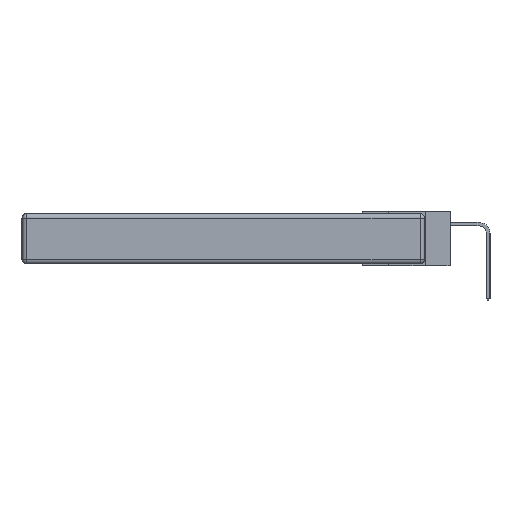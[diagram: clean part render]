
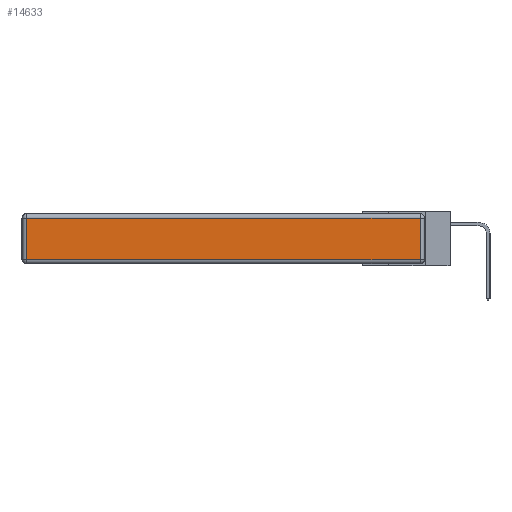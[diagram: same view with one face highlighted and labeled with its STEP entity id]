
A CAD part, left-side view. The second image highlights one B-rep face of the part: STEP entity #14633.
In plain terms, the highlighted planar face has unit normal (-1, 0, 0).
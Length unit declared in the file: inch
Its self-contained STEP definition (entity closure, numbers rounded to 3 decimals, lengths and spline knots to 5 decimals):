
#214 = VERTEX_POINT ( 'NONE', #12828 ) ;
#379 = VERTEX_POINT ( 'NONE', #14733 ) ;
#755 = CARTESIAN_POINT ( 'NONE',  ( 0., 0., -0.313 ) ) ;
#1602 = DIRECTION ( 'NONE',  ( 0., 0., 1. ) ) ;
#2339 = EDGE_CURVE ( 'NONE', #214, #11328, #6096, .T. ) ;
#2449 = ORIENTED_EDGE ( 'NONE', *, *, #2339, .T. ) ;
#4370 = ORIENTED_EDGE ( 'NONE', *, *, #13561, .T. ) ;
#4635 = CARTESIAN_POINT ( 'NONE',  ( 0., 2.75, -0.03 ) ) ;
#6096 = LINE ( 'NONE', #17140, #16647 ) ;
#6126 = DIRECTION ( 'NONE',  ( 0., 0., -1. ) ) ;
#6571 = EDGE_CURVE ( 'NONE', #11328, #15011, #13631, .T. ) ;
#7187 = LINE ( 'NONE', #755, #8609 ) ;
#8020 = LINE ( 'NONE', #10460, #13421 ) ;
#8609 = VECTOR ( 'NONE', #14174, 39.37008 ) ;
#8952 = PLANE ( 'NONE',  #14220 ) ;
#9054 = CARTESIAN_POINT ( 'NONE',  ( 0., 0.03, -0.03 ) ) ;
#9295 = FACE_OUTER_BOUND ( 'NONE', #10031, .T. ) ;
#9545 = DIRECTION ( 'NONE',  ( 0., 0., 1. ) ) ;
#10031 = EDGE_LOOP ( 'NONE', ( #4370, #2449, #17600, #19338 ) ) ;
#10460 = CARTESIAN_POINT ( 'NONE',  ( 0., 2.72, -0.343 ) ) ;
#11328 = VERTEX_POINT ( 'NONE', #9054 ) ;
#12049 = DIRECTION ( 'NONE',  ( -1., 0., 0. ) ) ;
#12061 = DIRECTION ( 'NONE',  ( 0., 1., 0. ) ) ;
#12828 = CARTESIAN_POINT ( 'NONE',  ( 0., 0.03, -0.313 ) ) ;
#13421 = VECTOR ( 'NONE', #6126, 39.37008 ) ;
#13492 = CARTESIAN_POINT ( 'NONE',  ( 0., 0., -0.343 ) ) ;
#13561 = EDGE_CURVE ( 'NONE', #379, #214, #7187, .T. ) ;
#13631 = LINE ( 'NONE', #4635, #16951 ) ;
#14174 = DIRECTION ( 'NONE',  ( 0., -1., 0. ) ) ;
#14220 = AXIS2_PLACEMENT_3D ( 'NONE', #13492, #12049, #1602 ) ;
#14633 = ADVANCED_FACE ( 'NONE', ( #9295 ), #8952, .T. ) ;
#14733 = CARTESIAN_POINT ( 'NONE',  ( 0., 2.72, -0.313 ) ) ;
#15011 = VERTEX_POINT ( 'NONE', #18201 ) ;
#16647 = VECTOR ( 'NONE', #9545, 39.37008 ) ;
#16951 = VECTOR ( 'NONE', #12061, 39.37008 ) ;
#17140 = CARTESIAN_POINT ( 'NONE',  ( 0., 0.03, -0.343 ) ) ;
#17600 = ORIENTED_EDGE ( 'NONE', *, *, #6571, .T. ) ;
#18201 = CARTESIAN_POINT ( 'NONE',  ( 0., 2.72, -0.03 ) ) ;
#19152 = EDGE_CURVE ( 'NONE', #15011, #379, #8020, .T. ) ;
#19338 = ORIENTED_EDGE ( 'NONE', *, *, #19152, .T. ) ;
